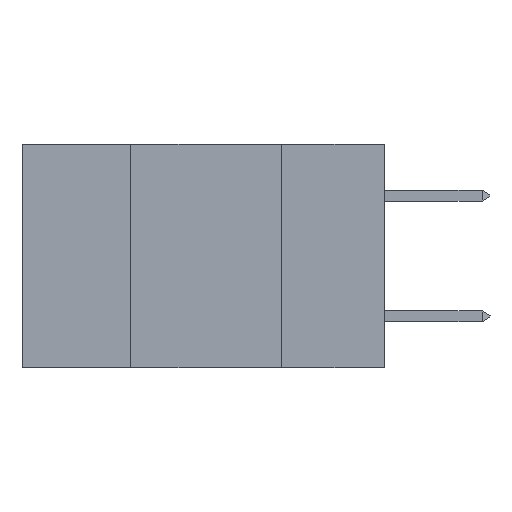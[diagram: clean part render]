
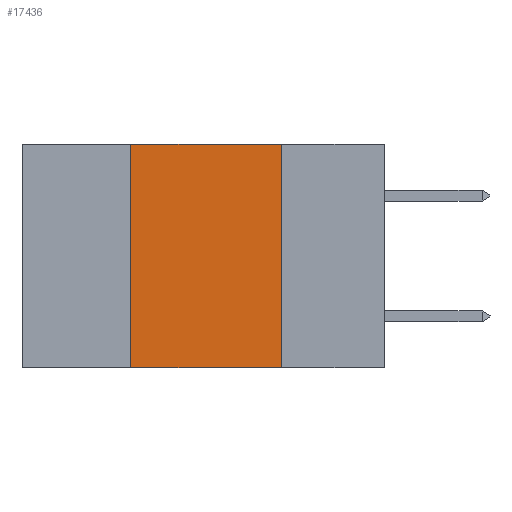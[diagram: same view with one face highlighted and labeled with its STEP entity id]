
A CAD part, left-side view. The second image highlights one B-rep face of the part: STEP entity #17436.
In plain terms, the highlighted planar face has unit normal (-1, 0, 0).
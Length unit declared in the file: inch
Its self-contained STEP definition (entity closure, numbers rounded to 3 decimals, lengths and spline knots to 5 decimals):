
#317 = VERTEX_POINT ( 'NONE', #10820 ) ;
#362 = EDGE_CURVE ( 'NONE', #317, #26573, #21391, .T. ) ;
#1613 = DIRECTION ( 'NONE',  ( 0., -1., 0. ) ) ;
#1886 = LINE ( 'NONE', #14800, #15270 ) ;
#2134 = LINE ( 'NONE', #14915, #2329 ) ;
#2329 = VECTOR ( 'NONE', #23514, 39.37008 ) ;
#3839 = FACE_OUTER_BOUND ( 'NONE', #21625, .T. ) ;
#3969 = VECTOR ( 'NONE', #25998, 39.37008 ) ;
#4901 = ORIENTED_EDGE ( 'NONE', *, *, #8488, .T. ) ;
#5832 = ORIENTED_EDGE ( 'NONE', *, *, #25203, .F. ) ;
#7473 = LINE ( 'NONE', #20288, #11589 ) ;
#8488 = EDGE_CURVE ( 'NONE', #11137, #21241, #1886, .T. ) ;
#10820 = CARTESIAN_POINT ( 'NONE',  ( 0., 0.42, 0. ) ) ;
#11137 = VERTEX_POINT ( 'NONE', #23334 ) ;
#11589 = VECTOR ( 'NONE', #14052, 39.37008 ) ;
#14052 = DIRECTION ( 'NONE',  ( 0., 0., -1. ) ) ;
#14800 = CARTESIAN_POINT ( 'NONE',  ( 0., 0.6, -0.37 ) ) ;
#14915 = CARTESIAN_POINT ( 'NONE',  ( 0., 0.42, 0. ) ) ;
#15270 = VECTOR ( 'NONE', #1613, 39.37008 ) ;
#17436 = ADVANCED_FACE ( 'NONE', ( #3839 ), #27459, .F. ) ;
#18629 = CARTESIAN_POINT ( 'NONE',  ( 0., 0.17, -0.37 ) ) ;
#19025 = EDGE_CURVE ( 'NONE', #26573, #21241, #7473, .T. ) ;
#20288 = CARTESIAN_POINT ( 'NONE',  ( 0., 0.17, 0. ) ) ;
#20465 = CARTESIAN_POINT ( 'NONE',  ( 0., 0.17, 0. ) ) ;
#20719 = CARTESIAN_POINT ( 'NONE',  ( 0., 0.6, 0. ) ) ;
#20855 = DIRECTION ( 'NONE',  ( 0., 0., -1. ) ) ;
#21241 = VERTEX_POINT ( 'NONE', #18629 ) ;
#21391 = LINE ( 'NONE', #27699, #3969 ) ;
#21625 = EDGE_LOOP ( 'NONE', ( #23637, #27139, #5832, #4901 ) ) ;
#23334 = CARTESIAN_POINT ( 'NONE',  ( 0., 0.42, -0.37 ) ) ;
#23514 = DIRECTION ( 'NONE',  ( 0., 0., 1. ) ) ;
#23637 = ORIENTED_EDGE ( 'NONE', *, *, #19025, .F. ) ;
#25203 = EDGE_CURVE ( 'NONE', #11137, #317, #2134, .T. ) ;
#25856 = AXIS2_PLACEMENT_3D ( 'NONE', #20719, #27177, #20855 ) ;
#25998 = DIRECTION ( 'NONE',  ( 0., -1., 0. ) ) ;
#26573 = VERTEX_POINT ( 'NONE', #20465 ) ;
#27139 = ORIENTED_EDGE ( 'NONE', *, *, #362, .F. ) ;
#27177 = DIRECTION ( 'NONE',  ( 1., 0., 0. ) ) ;
#27459 = PLANE ( 'NONE',  #25856 ) ;
#27699 = CARTESIAN_POINT ( 'NONE',  ( 0., 0.6, 0. ) ) ;
